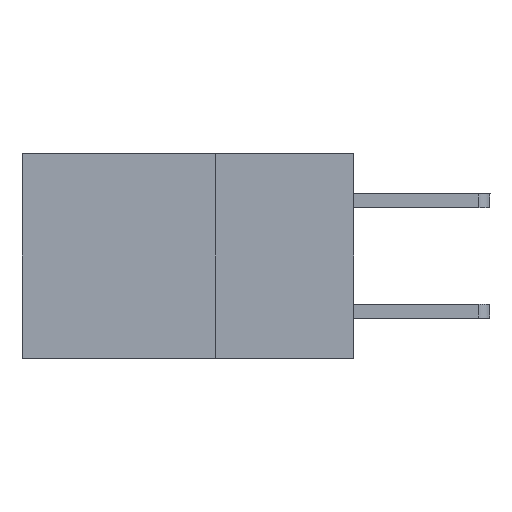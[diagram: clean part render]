
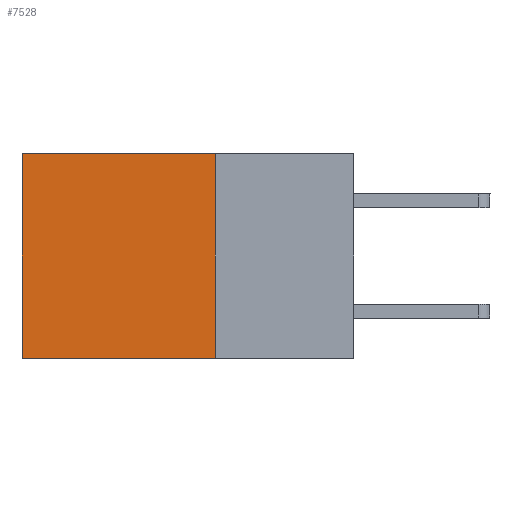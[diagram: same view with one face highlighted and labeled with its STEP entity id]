
A CAD part, left-side view. The second image highlights one B-rep face of the part: STEP entity #7528.
In plain terms, the highlighted planar face has unit normal (-1, 0, 0).
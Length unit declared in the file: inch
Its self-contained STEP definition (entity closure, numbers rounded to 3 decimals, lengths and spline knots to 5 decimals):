
#433 = EDGE_LOOP ( 'NONE', ( #543, #2129, #2249, #2289 ) ) ;
#520 = LINE ( 'NONE', #8709, #2374 ) ;
#543 = ORIENTED_EDGE ( 'NONE', *, *, #3425, .T. ) ;
#615 = DIRECTION ( 'NONE',  ( 0., 1., 0. ) ) ;
#999 = VERTEX_POINT ( 'NONE', #7803 ) ;
#1323 = LINE ( 'NONE', #4743, #3120 ) ;
#1622 = EDGE_CURVE ( 'NONE', #7272, #3556, #6089, .T. ) ;
#1667 = CARTESIAN_POINT ( 'NONE',  ( 0.2875, 0.6, -0.37 ) ) ;
#1935 = PLANE ( 'NONE',  #3475 ) ;
#2129 = ORIENTED_EDGE ( 'NONE', *, *, #1622, .F. ) ;
#2249 = ORIENTED_EDGE ( 'NONE', *, *, #6680, .F. ) ;
#2289 = ORIENTED_EDGE ( 'NONE', *, *, #6490, .T. ) ;
#2374 = VECTOR ( 'NONE', #615, 39.37008 ) ;
#2463 = CARTESIAN_POINT ( 'NONE',  ( 0.2875, 0.6, 0. ) ) ;
#2646 = DIRECTION ( 'NONE',  ( 1., 0., 0. ) ) ;
#2743 = DIRECTION ( 'NONE',  ( 0., 1., 0. ) ) ;
#3120 = VECTOR ( 'NONE', #5010, 39.37008 ) ;
#3184 = LINE ( 'NONE', #4440, #6934 ) ;
#3425 = EDGE_CURVE ( 'NONE', #8477, #3556, #1323, .T. ) ;
#3475 = AXIS2_PLACEMENT_3D ( 'NONE', #8481, #2646, #7837 ) ;
#3556 = VERTEX_POINT ( 'NONE', #1667 ) ;
#3988 = CARTESIAN_POINT ( 'NONE',  ( 0.2875, 0.25, -0.37 ) ) ;
#4440 = CARTESIAN_POINT ( 'NONE',  ( 0.2875, 0.25, 0. ) ) ;
#4516 = DIRECTION ( 'NONE',  ( 0., 0., -1. ) ) ;
#4743 = CARTESIAN_POINT ( 'NONE',  ( 0.2875, 0.6, 0. ) ) ;
#5010 = DIRECTION ( 'NONE',  ( 0., 0., -1. ) ) ;
#5387 = CARTESIAN_POINT ( 'NONE',  ( 0.2875, 0.25, -0.37 ) ) ;
#5841 = VECTOR ( 'NONE', #2743, 39.37008 ) ;
#6089 = LINE ( 'NONE', #5387, #5841 ) ;
#6490 = EDGE_CURVE ( 'NONE', #999, #8477, #520, .T. ) ;
#6680 = EDGE_CURVE ( 'NONE', #999, #7272, #3184, .T. ) ;
#6934 = VECTOR ( 'NONE', #4516, 39.37008 ) ;
#7272 = VERTEX_POINT ( 'NONE', #3988 ) ;
#7528 = ADVANCED_FACE ( 'NONE', ( #8862 ), #1935, .F. ) ;
#7803 = CARTESIAN_POINT ( 'NONE',  ( 0.2875, 0.25, 0. ) ) ;
#7837 = DIRECTION ( 'NONE',  ( 0., 0., -1. ) ) ;
#8477 = VERTEX_POINT ( 'NONE', #2463 ) ;
#8481 = CARTESIAN_POINT ( 'NONE',  ( 0.2875, 0.25, 0. ) ) ;
#8709 = CARTESIAN_POINT ( 'NONE',  ( 0.2875, 0.25, 0. ) ) ;
#8862 = FACE_OUTER_BOUND ( 'NONE', #433, .T. ) ;
